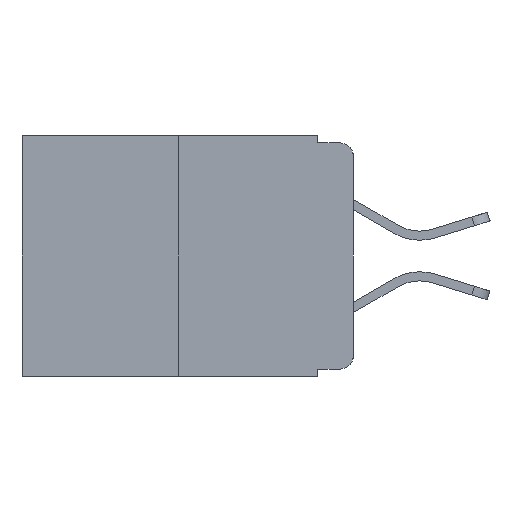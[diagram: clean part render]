
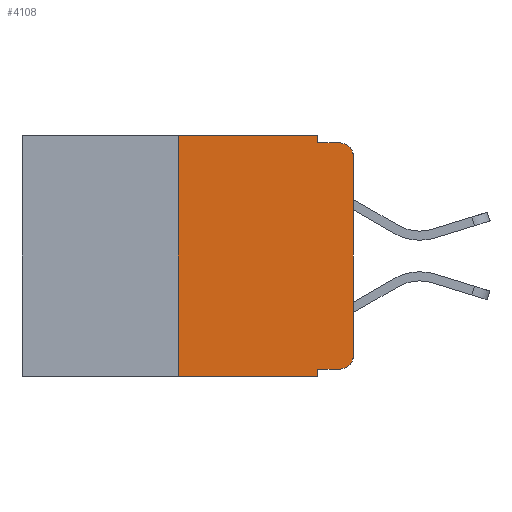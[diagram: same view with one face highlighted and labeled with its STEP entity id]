
A CAD part, left-side view. The second image highlights one B-rep face of the part: STEP entity #4108.
In plain terms, the highlighted planar face has unit normal (-1, 0, 0).
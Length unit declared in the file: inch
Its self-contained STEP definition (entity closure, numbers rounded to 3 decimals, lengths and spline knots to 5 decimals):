
#236 = CARTESIAN_POINT ( 'NONE',  ( 0., 0.25, 0. ) ) ;
#367 = EDGE_CURVE ( 'NONE', #803, #6483, #6015, .T. ) ;
#803 = VERTEX_POINT ( 'NONE', #9330 ) ;
#813 = DIRECTION ( 'NONE',  ( 0., -1., 0. ) ) ;
#1162 = CARTESIAN_POINT ( 'NONE',  ( 0., 0.02, -0.03 ) ) ;
#1337 = CARTESIAN_POINT ( 'NONE',  ( 0., 0.25, 0. ) ) ;
#1733 = ORIENTED_EDGE ( 'NONE', *, *, #6058, .T. ) ;
#1826 = ORIENTED_EDGE ( 'NONE', *, *, #11105, .F. ) ;
#2102 = EDGE_CURVE ( 'NONE', #4811, #4621, #10017, .T. ) ;
#2215 = CARTESIAN_POINT ( 'NONE',  ( 0., 0.051, 0. ) ) ;
#2264 = DIRECTION ( 'NONE',  ( 0., 0., -1. ) ) ;
#2527 = DIRECTION ( 'NONE',  ( 0., 0., -1. ) ) ;
#2634 = ORIENTED_EDGE ( 'NONE', *, *, #367, .F. ) ;
#3385 = AXIS2_PLACEMENT_3D ( 'NONE', #1162, #8229, #2264 ) ;
#3398 = ORIENTED_EDGE ( 'NONE', *, *, #10548, .T. ) ;
#3449 = DIRECTION ( 'NONE',  ( 0., -1., 0. ) ) ;
#3455 = CIRCLE ( 'NONE', #3385, 0.02 ) ;
#3474 = CIRCLE ( 'NONE', #4383, 0.02 ) ;
#3509 = PLANE ( 'NONE',  #11525 ) ;
#3555 = CARTESIAN_POINT ( 'NONE',  ( 0., 0.02, -0.333 ) ) ;
#3572 = CARTESIAN_POINT ( 'NONE',  ( 0., 0.473, 0. ) ) ;
#3847 = ORIENTED_EDGE ( 'NONE', *, *, #7108, .T. ) ;
#3906 = LINE ( 'NONE', #2215, #6304 ) ;
#4108 = ADVANCED_FACE ( 'NONE', ( #8739 ), #3509, .F. ) ;
#4363 = ORIENTED_EDGE ( 'NONE', *, *, #4702, .F. ) ;
#4383 = AXIS2_PLACEMENT_3D ( 'NONE', #5492, #11817, #6496 ) ;
#4519 = CARTESIAN_POINT ( 'NONE',  ( 0., 0.473, -0.343 ) ) ;
#4549 = ORIENTED_EDGE ( 'NONE', *, *, #9088, .T. ) ;
#4621 = VERTEX_POINT ( 'NONE', #8114 ) ;
#4702 = EDGE_CURVE ( 'NONE', #4621, #803, #9275, .T. ) ;
#4811 = VERTEX_POINT ( 'NONE', #1337 ) ;
#5012 = VECTOR ( 'NONE', #6396, 39.37008 ) ;
#5213 = LINE ( 'NONE', #236, #9357 ) ;
#5280 = CARTESIAN_POINT ( 'NONE',  ( 0., 0., -0.313 ) ) ;
#5492 = CARTESIAN_POINT ( 'NONE',  ( 0., 0.02, -0.313 ) ) ;
#5570 = VECTOR ( 'NONE', #7500, 39.37008 ) ;
#5698 = VECTOR ( 'NONE', #3449, 39.37008 ) ;
#5809 = ORIENTED_EDGE ( 'NONE', *, *, #11683, .F. ) ;
#5864 = EDGE_LOOP ( 'NONE', ( #3847, #1733, #2634, #4363, #6761, #1826, #7073, #5809, #3398, #4549 ) ) ;
#6015 = LINE ( 'NONE', #6873, #5698 ) ;
#6049 = CARTESIAN_POINT ( 'NONE',  ( 0., 0.02, -0.01 ) ) ;
#6058 = EDGE_CURVE ( 'NONE', #6361, #6483, #3455, .T. ) ;
#6220 = VERTEX_POINT ( 'NONE', #3555 ) ;
#6304 = VECTOR ( 'NONE', #12514, 39.37008 ) ;
#6361 = VERTEX_POINT ( 'NONE', #11264 ) ;
#6374 = VERTEX_POINT ( 'NONE', #6907 ) ;
#6396 = DIRECTION ( 'NONE',  ( 0., -1., 0. ) ) ;
#6483 = VERTEX_POINT ( 'NONE', #6049 ) ;
#6496 = DIRECTION ( 'NONE',  ( 0., 0., -1. ) ) ;
#6638 = VECTOR ( 'NONE', #813, 39.37008 ) ;
#6761 = ORIENTED_EDGE ( 'NONE', *, *, #2102, .F. ) ;
#6873 = CARTESIAN_POINT ( 'NONE',  ( 0., 0.051, -0.01 ) ) ;
#6907 = CARTESIAN_POINT ( 'NONE',  ( 0., 0.051, -0.333 ) ) ;
#7024 = CARTESIAN_POINT ( 'NONE',  ( 0., 0.051, -0.333 ) ) ;
#7073 = ORIENTED_EDGE ( 'NONE', *, *, #9155, .T. ) ;
#7108 = EDGE_CURVE ( 'NONE', #7923, #6361, #9822, .T. ) ;
#7291 = DIRECTION ( 'NONE',  ( 0., 0., -1. ) ) ;
#7424 = VECTOR ( 'NONE', #11614, 39.37008 ) ;
#7500 = DIRECTION ( 'NONE',  ( 0., -1., 0. ) ) ;
#7693 = CARTESIAN_POINT ( 'NONE',  ( 0., 0.25, -0.343 ) ) ;
#7923 = VERTEX_POINT ( 'NONE', #5280 ) ;
#8114 = CARTESIAN_POINT ( 'NONE',  ( 0., 0.051, 0. ) ) ;
#8144 = LINE ( 'NONE', #4519, #5570 ) ;
#8190 = VERTEX_POINT ( 'NONE', #11003 ) ;
#8229 = DIRECTION ( 'NONE',  ( -1., 0., 0. ) ) ;
#8477 = DIRECTION ( 'NONE',  ( 0., 0., 1. ) ) ;
#8739 = FACE_OUTER_BOUND ( 'NONE', #5864, .T. ) ;
#8962 = CARTESIAN_POINT ( 'NONE',  ( 0., 0.473, 0. ) ) ;
#9088 = EDGE_CURVE ( 'NONE', #6220, #7923, #3474, .T. ) ;
#9092 = LINE ( 'NONE', #7024, #6638 ) ;
#9155 = EDGE_CURVE ( 'NONE', #10272, #8190, #8144, .T. ) ;
#9275 = LINE ( 'NONE', #11649, #10999 ) ;
#9330 = CARTESIAN_POINT ( 'NONE',  ( 0., 0.051, -0.01 ) ) ;
#9357 = VECTOR ( 'NONE', #8477, 39.37008 ) ;
#9822 = LINE ( 'NONE', #9930, #7424 ) ;
#9930 = CARTESIAN_POINT ( 'NONE',  ( 0., 0., 0. ) ) ;
#10017 = LINE ( 'NONE', #8962, #5012 ) ;
#10272 = VERTEX_POINT ( 'NONE', #7693 ) ;
#10548 = EDGE_CURVE ( 'NONE', #6374, #6220, #9092, .T. ) ;
#10999 = VECTOR ( 'NONE', #7291, 39.37008 ) ;
#11003 = CARTESIAN_POINT ( 'NONE',  ( 0., 0.051, -0.343 ) ) ;
#11105 = EDGE_CURVE ( 'NONE', #10272, #4811, #5213, .T. ) ;
#11264 = CARTESIAN_POINT ( 'NONE',  ( 0., 0., -0.03 ) ) ;
#11525 = AXIS2_PLACEMENT_3D ( 'NONE', #3572, #11933, #2527 ) ;
#11614 = DIRECTION ( 'NONE',  ( 0., 0., 1. ) ) ;
#11649 = CARTESIAN_POINT ( 'NONE',  ( 0., 0.051, 0. ) ) ;
#11683 = EDGE_CURVE ( 'NONE', #6374, #8190, #3906, .T. ) ;
#11817 = DIRECTION ( 'NONE',  ( -1., 0., 0. ) ) ;
#11933 = DIRECTION ( 'NONE',  ( 1., 0., 0. ) ) ;
#12514 = DIRECTION ( 'NONE',  ( 0., 0., -1. ) ) ;
